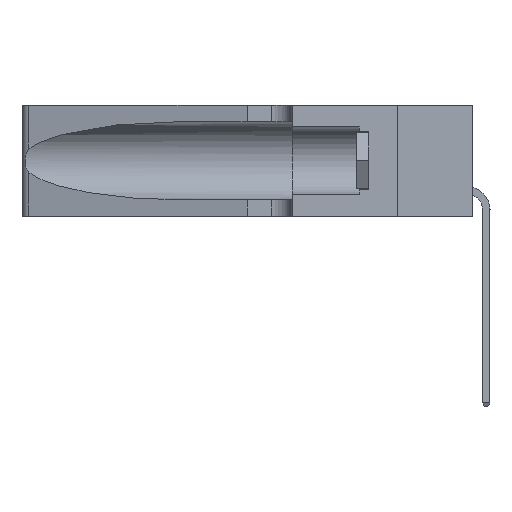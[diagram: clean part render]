
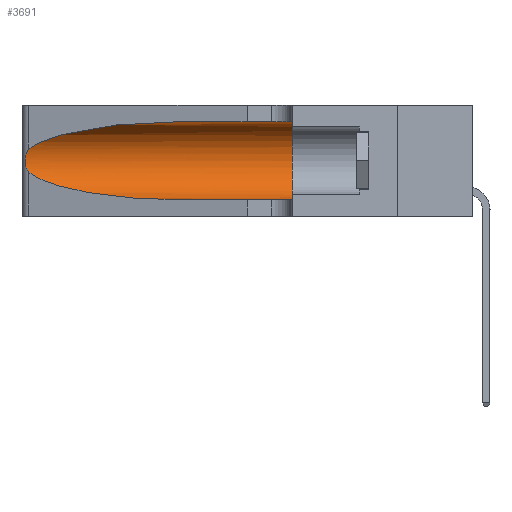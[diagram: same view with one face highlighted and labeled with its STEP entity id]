
A CAD part, left-side view. The second image highlights one B-rep face of the part: STEP entity #3691.
In plain terms, the highlighted cylindrical face has radius 3.308 mm (diameter 6.617 mm), a partial arc.
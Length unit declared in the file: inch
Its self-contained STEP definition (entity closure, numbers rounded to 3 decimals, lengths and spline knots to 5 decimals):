
#46 = CARTESIAN_POINT ( 'NONE',  ( 0.1305, 1.61858, 0.31525 ) ) ;
#130 = CARTESIAN_POINT ( 'NONE',  ( 0.1305, 0.35, 0.31525 ) ) ;
#594 = EDGE_CURVE ( 'NONE', #11257, #19204, #3675, .T. ) ;
#1221 = CARTESIAN_POINT ( 'NONE',  ( 0.25555, 1.22993, 0.14849 ) ) ;
#1972 = CARTESIAN_POINT ( 'NONE',  ( 0.18966, 0.96281, 0.31525 ) ) ;
#1997 = EDGE_LOOP ( 'NONE', ( #5860, #11327, #19072, #7292, #18167, #10322 ) ) ;
#2039 = CYLINDRICAL_SURFACE ( 'NONE', #19558, 0.13025 ) ;
#2392 = EDGE_CURVE ( 'NONE', #19204, #5205, #9307, .T. ) ;
#3119 =( BOUNDED_CURVE ( )  B_SPLINE_CURVE ( 3, ( #15351, #1972, #18336, #18542 ),
 .UNSPECIFIED., .F., .F. ) 
 B_SPLINE_CURVE_WITH_KNOTS ( ( 4, 4 ),
 ( 1.5708, 2.84003 ),
 .UNSPECIFIED. ) 
 CURVE ( )  GEOMETRIC_REPRESENTATION_ITEM ( )  RATIONAL_B_SPLINE_CURVE ( ( 1., 0.87, 0.87, 1. ) ) 
 REPRESENTATION_ITEM ( '' )  );
#3125 = AXIS2_PLACEMENT_3D ( 'NONE', #17018, #18340, #15361 ) ;
#3675 = LINE ( 'NONE', #46, #4854 ) ;
#3691 = ADVANCED_FACE ( 'NONE', ( #6008 ), #2039, .F. ) ;
#3880 = EDGE_CURVE ( 'NONE', #11257, #7597, #3119, .T. ) ;
#4217 = CARTESIAN_POINT ( 'NONE',  ( 0.26075, 1.23896, 0.19203 ) ) ;
#4473 = EDGE_CURVE ( 'NONE', #15002, #5205, #12467, .T. ) ;
#4564 =( BOUNDED_CURVE ( )  B_SPLINE_CURVE ( 3, ( #18074, #8988, #10528, #11726 ),
 .UNSPECIFIED., .F., .T. ) 
 B_SPLINE_CURVE_WITH_KNOTS ( ( 4, 4 ),
 ( 3.44316, 4.71239 ),
 .UNSPECIFIED. ) 
 CURVE ( )  GEOMETRIC_REPRESENTATION_ITEM ( )  RATIONAL_B_SPLINE_CURVE ( ( 1., 0.87, 0.87, 1. ) ) 
 REPRESENTATION_ITEM ( '' )  );
#4854 = VECTOR ( 'NONE', #11697, 39.37008 ) ;
#5205 = VERTEX_POINT ( 'NONE', #12503 ) ;
#5725 = CARTESIAN_POINT ( 'NONE',  ( 0.26017, 1.23833, 0.17102 ) ) ;
#5860 = ORIENTED_EDGE ( 'NONE', *, *, #3880, .T. ) ;
#5905 = EDGE_CURVE ( 'NONE', #7597, #18056, #12876, .T. ) ;
#6008 = FACE_OUTER_BOUND ( 'NONE', #1997, .T. ) ;
#6322 = DIRECTION ( 'NONE',  ( 0., -1., 0. ) ) ;
#6897 = EDGE_CURVE ( 'NONE', #18056, #15002, #4564, .T. ) ;
#7224 = CARTESIAN_POINT ( 'NONE',  ( 0.1305, 0.72297, 0.05475 ) ) ;
#7262 = CARTESIAN_POINT ( 'NONE',  ( 0.26018, 1.23835, 0.19895 ) ) ;
#7292 = ORIENTED_EDGE ( 'NONE', *, *, #4473, .T. ) ;
#7597 = VERTEX_POINT ( 'NONE', #16774 ) ;
#8988 = CARTESIAN_POINT ( 'NONE',  ( 0.2373, 1.15595, 0.08982 ) ) ;
#9159 = CARTESIAN_POINT ( 'NONE',  ( 0.25854, 1.2359, 0.20912 ) ) ;
#9307 = CIRCLE ( 'NONE', #3125, 0.13025 ) ;
#10322 = ORIENTED_EDGE ( 'NONE', *, *, #594, .F. ) ;
#10354 = CARTESIAN_POINT ( 'NONE',  ( 0.25789, 1.23486, 0.15765 ) ) ;
#10528 = CARTESIAN_POINT ( 'NONE',  ( 0.18966, 0.96281, 0.05475 ) ) ;
#10707 = CARTESIAN_POINT ( 'NONE',  ( 0.25856, 1.23593, 0.16098 ) ) ;
#11257 = VERTEX_POINT ( 'NONE', #18046 ) ;
#11327 = ORIENTED_EDGE ( 'NONE', *, *, #5905, .T. ) ;
#11697 = DIRECTION ( 'NONE',  ( 0., -1., 0. ) ) ;
#11726 = CARTESIAN_POINT ( 'NONE',  ( 0.1305, 0.72297, 0.05475 ) ) ;
#11814 = CARTESIAN_POINT ( 'NONE',  ( 0.25787, 1.23484, 0.2124 ) ) ;
#12016 = DIRECTION ( 'NONE',  ( 0., -1., 0. ) ) ;
#12467 = LINE ( 'NONE', #18556, #19571 ) ;
#12503 = CARTESIAN_POINT ( 'NONE',  ( 0.1305, 0.35, 0.05475 ) ) ;
#12876 = B_SPLINE_CURVE_WITH_KNOTS ( 'NONE', 3,
 ( #16843, #19454, #14834, #11814, #9159, #7262, #4217, #18368, #5725, #10707, #10354, #17839, #1221, #19384 ),
 .UNSPECIFIED., .F., .F.,
 ( 4, 2, 2, 2, 2, 2, 4 ),
 ( 0., 0.00027, 0.00053, 0.00107, 0.0016, 0.00187, 0.00214 ),
 .UNSPECIFIED. ) ;
#13350 = DIRECTION ( 'NONE',  ( 0., 0., -1. ) ) ;
#14834 = CARTESIAN_POINT ( 'NONE',  ( 0.25639, 1.23184, 0.21858 ) ) ;
#15002 = VERTEX_POINT ( 'NONE', #7224 ) ;
#15351 = CARTESIAN_POINT ( 'NONE',  ( 0.1305, 0.72297, 0.31525 ) ) ;
#15361 = DIRECTION ( 'NONE',  ( 0., 0., 1. ) ) ;
#16574 = CARTESIAN_POINT ( 'NONE',  ( 0.1305, 1.61858, 0.185 ) ) ;
#16774 = CARTESIAN_POINT ( 'NONE',  ( 0.25487, 1.22718, 0.22369 ) ) ;
#16843 = CARTESIAN_POINT ( 'NONE',  ( 0.25487, 1.22718, 0.22369 ) ) ;
#17018 = CARTESIAN_POINT ( 'NONE',  ( 0.1305, 0.35, 0.185 ) ) ;
#17350 = CARTESIAN_POINT ( 'NONE',  ( 0.25487, 1.22718, 0.14631 ) ) ;
#17839 = CARTESIAN_POINT ( 'NONE',  ( 0.25639, 1.23186, 0.15144 ) ) ;
#18046 = CARTESIAN_POINT ( 'NONE',  ( 0.1305, 0.72297, 0.31525 ) ) ;
#18056 = VERTEX_POINT ( 'NONE', #17350 ) ;
#18074 = CARTESIAN_POINT ( 'NONE',  ( 0.25487, 1.22718, 0.14631 ) ) ;
#18167 = ORIENTED_EDGE ( 'NONE', *, *, #2392, .F. ) ;
#18336 = CARTESIAN_POINT ( 'NONE',  ( 0.2373, 1.15595, 0.28018 ) ) ;
#18340 = DIRECTION ( 'NONE',  ( 0., 1., 0. ) ) ;
#18368 = CARTESIAN_POINT ( 'NONE',  ( 0.26075, 1.23896, 0.178 ) ) ;
#18542 = CARTESIAN_POINT ( 'NONE',  ( 0.25487, 1.22718, 0.22369 ) ) ;
#18556 = CARTESIAN_POINT ( 'NONE',  ( 0.1305, 1.61858, 0.05475 ) ) ;
#19072 = ORIENTED_EDGE ( 'NONE', *, *, #6897, .T. ) ;
#19204 = VERTEX_POINT ( 'NONE', #130 ) ;
#19384 = CARTESIAN_POINT ( 'NONE',  ( 0.25487, 1.22718, 0.14631 ) ) ;
#19454 = CARTESIAN_POINT ( 'NONE',  ( 0.25555, 1.22994, 0.2215 ) ) ;
#19558 = AXIS2_PLACEMENT_3D ( 'NONE', #16574, #12016, #13350 ) ;
#19571 = VECTOR ( 'NONE', #6322, 39.37008 ) ;
